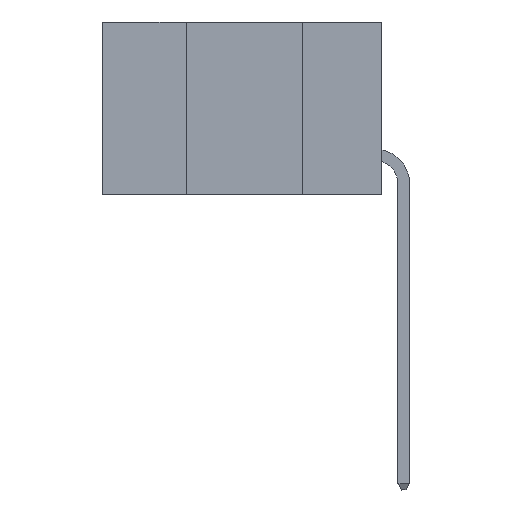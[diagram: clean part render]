
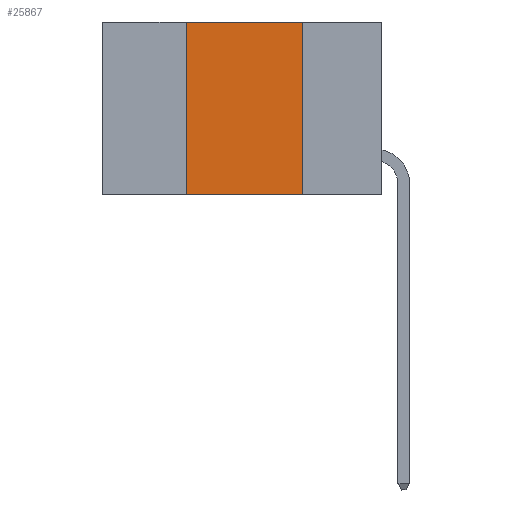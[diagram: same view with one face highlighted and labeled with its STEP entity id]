
A CAD part, left-side view. The second image highlights one B-rep face of the part: STEP entity #25867.
In plain terms, the highlighted planar face has unit normal (-1, 0, 0).
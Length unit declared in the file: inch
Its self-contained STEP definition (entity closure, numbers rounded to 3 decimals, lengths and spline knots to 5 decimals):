
#70 = LINE ( 'NONE', #31236, #4228 ) ;
#231 = ORIENTED_EDGE ( 'NONE', *, *, #32467, .F. ) ;
#1173 = ORIENTED_EDGE ( 'NONE', *, *, #23695, .F. ) ;
#3364 = LINE ( 'NONE', #30157, #34103 ) ;
#3772 = VECTOR ( 'NONE', #18288, 39.37008 ) ;
#4228 = VECTOR ( 'NONE', #13430, 39.37008 ) ;
#5506 = VECTOR ( 'NONE', #8531, 39.37008 ) ;
#6234 = DIRECTION ( 'NONE',  ( 0., 0., -1. ) ) ;
#8531 = DIRECTION ( 'NONE',  ( 0., -1., 0. ) ) ;
#10878 = VERTEX_POINT ( 'NONE', #37688 ) ;
#11518 = CARTESIAN_POINT ( 'NONE',  ( 0., 0.6, 0. ) ) ;
#11626 = EDGE_LOOP ( 'NONE', ( #1173, #29124, #231, #26271 ) ) ;
#13430 = DIRECTION ( 'NONE',  ( 0., 0., 1. ) ) ;
#13454 = LINE ( 'NONE', #11518, #5506 ) ;
#14436 = CARTESIAN_POINT ( 'NONE',  ( 0., 0.42, -0.37 ) ) ;
#14983 = LINE ( 'NONE', #29989, #3772 ) ;
#17616 = VERTEX_POINT ( 'NONE', #22683 ) ;
#18288 = DIRECTION ( 'NONE',  ( 0., -1., 0. ) ) ;
#22683 = CARTESIAN_POINT ( 'NONE',  ( 0., 0.17, -0.37 ) ) ;
#23695 = EDGE_CURVE ( 'NONE', #34770, #17616, #3364, .T. ) ;
#24332 = EDGE_CURVE ( 'NONE', #34792, #17616, #14983, .T. ) ;
#25867 = ADVANCED_FACE ( 'NONE', ( #33469 ), #28053, .F. ) ;
#26012 = EDGE_CURVE ( 'NONE', #10878, #34770, #13454, .T. ) ;
#26271 = ORIENTED_EDGE ( 'NONE', *, *, #24332, .T. ) ;
#28053 = PLANE ( 'NONE',  #36468 ) ;
#29124 = ORIENTED_EDGE ( 'NONE', *, *, #26012, .F. ) ;
#29215 = CARTESIAN_POINT ( 'NONE',  ( 0., 0.6, 0. ) ) ;
#29989 = CARTESIAN_POINT ( 'NONE',  ( 0., 0.6, -0.37 ) ) ;
#30157 = CARTESIAN_POINT ( 'NONE',  ( 0., 0.17, 0. ) ) ;
#31236 = CARTESIAN_POINT ( 'NONE',  ( 0., 0.42, 0. ) ) ;
#32467 = EDGE_CURVE ( 'NONE', #34792, #10878, #70, .T. ) ;
#33469 = FACE_OUTER_BOUND ( 'NONE', #11626, .T. ) ;
#34103 = VECTOR ( 'NONE', #6234, 39.37008 ) ;
#34659 = DIRECTION ( 'NONE',  ( 0., 0., -1. ) ) ;
#34770 = VERTEX_POINT ( 'NONE', #38497 ) ;
#34792 = VERTEX_POINT ( 'NONE', #14436 ) ;
#36468 = AXIS2_PLACEMENT_3D ( 'NONE', #29215, #38072, #34659 ) ;
#37688 = CARTESIAN_POINT ( 'NONE',  ( 0., 0.42, 0. ) ) ;
#38072 = DIRECTION ( 'NONE',  ( 1., 0., 0. ) ) ;
#38497 = CARTESIAN_POINT ( 'NONE',  ( 0., 0.17, 0. ) ) ;
